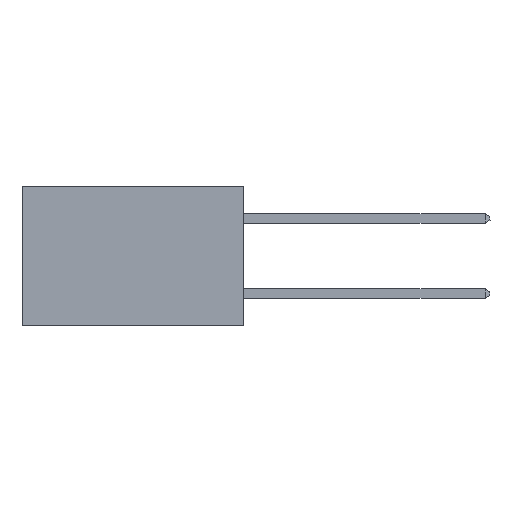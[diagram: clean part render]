
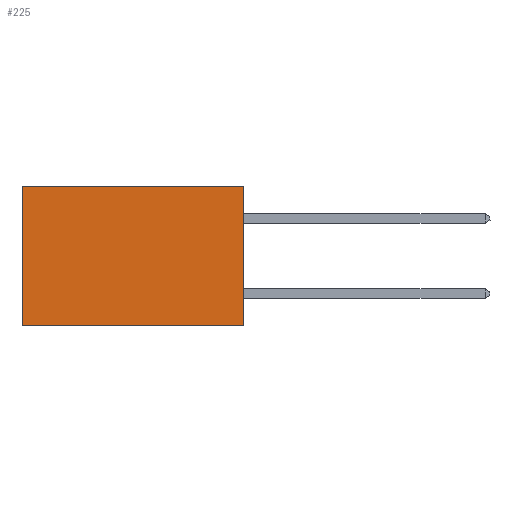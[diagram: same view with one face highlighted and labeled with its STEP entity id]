
A CAD part, left-side view. The second image highlights one B-rep face of the part: STEP entity #225.
In plain terms, the highlighted planar face has unit normal (-1, 0, 0).
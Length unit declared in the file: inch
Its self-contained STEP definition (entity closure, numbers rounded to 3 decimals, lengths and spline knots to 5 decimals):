
#225 = ADVANCED_FACE ( 'NONE', ( #7047 ), #6579, .F. ) ;
#471 = ORIENTED_EDGE ( 'NONE', *, *, #9113, .T. ) ;
#733 = VECTOR ( 'NONE', #6715, 39.37008 ) ;
#1013 = CARTESIAN_POINT ( 'NONE',  ( 0.277, 0.59, 0. ) ) ;
#1298 = CARTESIAN_POINT ( 'NONE',  ( 0.277, 0., -0.37 ) ) ;
#1473 = VECTOR ( 'NONE', #6697, 39.37008 ) ;
#1650 = ORIENTED_EDGE ( 'NONE', *, *, #7770, .F. ) ;
#1914 = LINE ( 'NONE', #2517, #9920 ) ;
#2337 = DIRECTION ( 'NONE',  ( 0., 0., -1. ) ) ;
#2517 = CARTESIAN_POINT ( 'NONE',  ( 0.277, 0., -0.37 ) ) ;
#2553 = DIRECTION ( 'NONE',  ( 0., 0., -1. ) ) ;
#2851 = ORIENTED_EDGE ( 'NONE', *, *, #7850, .F. ) ;
#2907 = CARTESIAN_POINT ( 'NONE',  ( 0.277, 0., -0.37 ) ) ;
#2933 = DIRECTION ( 'NONE',  ( 0., 1., 0. ) ) ;
#3150 = CARTESIAN_POINT ( 'NONE',  ( 0.277, 0., 0. ) ) ;
#3202 = VERTEX_POINT ( 'NONE', #1298 ) ;
#3695 = ORIENTED_EDGE ( 'NONE', *, *, #6778, .T. ) ;
#4623 = EDGE_LOOP ( 'NONE', ( #3695, #1650, #2851, #471 ) ) ;
#4678 = VERTEX_POINT ( 'NONE', #9623 ) ;
#4853 = VECTOR ( 'NONE', #2933, 39.37008 ) ;
#5809 = CARTESIAN_POINT ( 'NONE',  ( 0.277, 0., -0.37 ) ) ;
#6579 = PLANE ( 'NONE',  #6858 ) ;
#6697 = DIRECTION ( 'NONE',  ( 0., 1., 0. ) ) ;
#6715 = DIRECTION ( 'NONE',  ( 0., 0., -1. ) ) ;
#6758 = CARTESIAN_POINT ( 'NONE',  ( 0.277, 0.59, -0.37 ) ) ;
#6778 = EDGE_CURVE ( 'NONE', #9701, #4678, #7413, .T. ) ;
#6785 = CARTESIAN_POINT ( 'NONE',  ( 0.277, 0., 0. ) ) ;
#6858 = AXIS2_PLACEMENT_3D ( 'NONE', #5809, #9049, #2337 ) ;
#7047 = FACE_OUTER_BOUND ( 'NONE', #4623, .T. ) ;
#7168 = LINE ( 'NONE', #2907, #4853 ) ;
#7413 = LINE ( 'NONE', #6758, #733 ) ;
#7708 = VERTEX_POINT ( 'NONE', #3150 ) ;
#7770 = EDGE_CURVE ( 'NONE', #3202, #4678, #7168, .T. ) ;
#7850 = EDGE_CURVE ( 'NONE', #7708, #3202, #1914, .T. ) ;
#9049 = DIRECTION ( 'NONE',  ( 1., 0., 0. ) ) ;
#9113 = EDGE_CURVE ( 'NONE', #7708, #9701, #9777, .T. ) ;
#9623 = CARTESIAN_POINT ( 'NONE',  ( 0.277, 0.59, -0.37 ) ) ;
#9701 = VERTEX_POINT ( 'NONE', #1013 ) ;
#9777 = LINE ( 'NONE', #6785, #1473 ) ;
#9920 = VECTOR ( 'NONE', #2553, 39.37008 ) ;
